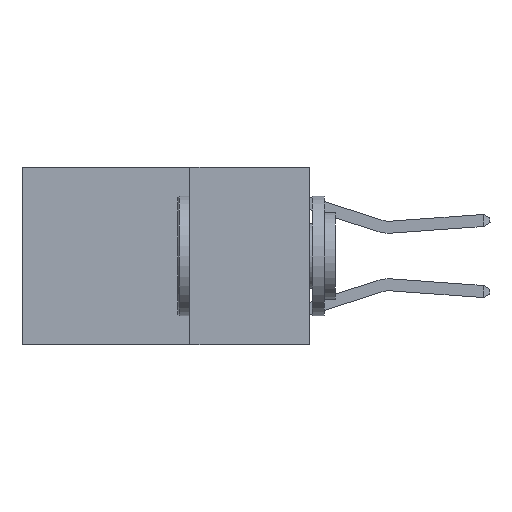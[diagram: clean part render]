
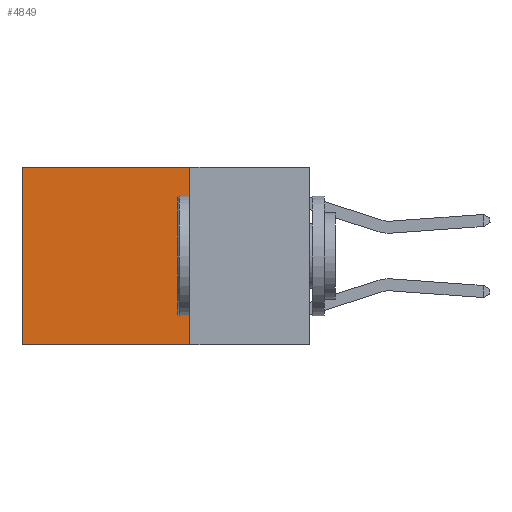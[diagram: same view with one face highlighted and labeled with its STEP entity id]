
A CAD part, left-side view. The second image highlights one B-rep face of the part: STEP entity #4849.
In plain terms, the highlighted planar face has unit normal (-1, 0, 0).
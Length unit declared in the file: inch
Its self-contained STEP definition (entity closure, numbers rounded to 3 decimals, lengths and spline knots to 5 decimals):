
#658 = VERTEX_POINT ( 'NONE', #7262 ) ;
#970 = VECTOR ( 'NONE', #3664, 39.37008 ) ;
#1154 = LINE ( 'NONE', #10167, #5738 ) ;
#1209 = VERTEX_POINT ( 'NONE', #4398 ) ;
#2331 = CARTESIAN_POINT ( 'NONE',  ( 0.2625, 0.25, 0. ) ) ;
#2369 = EDGE_CURVE ( 'NONE', #1209, #5428, #4144, .T. ) ;
#2580 = ORIENTED_EDGE ( 'NONE', *, *, #2369, .T. ) ;
#2636 = ORIENTED_EDGE ( 'NONE', *, *, #9742, .F. ) ;
#2655 = ORIENTED_EDGE ( 'NONE', *, *, #6685, .F. ) ;
#2946 = VERTEX_POINT ( 'NONE', #5557 ) ;
#2949 = ORIENTED_EDGE ( 'NONE', *, *, #4007, .T. ) ;
#3043 = CARTESIAN_POINT ( 'NONE',  ( 0.2625, 0.6, 0. ) ) ;
#3251 = PLANE ( 'NONE',  #6330 ) ;
#3318 = FACE_OUTER_BOUND ( 'NONE', #9757, .T. ) ;
#3664 = DIRECTION ( 'NONE',  ( 0., 0., -1. ) ) ;
#4007 = EDGE_CURVE ( 'NONE', #5428, #2946, #6175, .T. ) ;
#4144 = LINE ( 'NONE', #5724, #9201 ) ;
#4244 = CARTESIAN_POINT ( 'NONE',  ( 0.2625, 0.25, 0. ) ) ;
#4398 = CARTESIAN_POINT ( 'NONE',  ( 0.2625, 0.25, 0. ) ) ;
#4849 = ADVANCED_FACE ( 'NONE', ( #3318 ), #3251, .F. ) ;
#5181 = DIRECTION ( 'NONE',  ( 1., 0., 0. ) ) ;
#5428 = VERTEX_POINT ( 'NONE', #3043 ) ;
#5557 = CARTESIAN_POINT ( 'NONE',  ( 0.2625, 0.6, -0.37 ) ) ;
#5724 = CARTESIAN_POINT ( 'NONE',  ( 0.2625, 0.25, 0. ) ) ;
#5738 = VECTOR ( 'NONE', #10985, 39.37008 ) ;
#6175 = LINE ( 'NONE', #11529, #970 ) ;
#6235 = DIRECTION ( 'NONE',  ( 0., 0., -1. ) ) ;
#6264 = VECTOR ( 'NONE', #6235, 39.37008 ) ;
#6330 = AXIS2_PLACEMENT_3D ( 'NONE', #4244, #5181, #11194 ) ;
#6685 = EDGE_CURVE ( 'NONE', #658, #2946, #1154, .T. ) ;
#7262 = CARTESIAN_POINT ( 'NONE',  ( 0.2625, 0.25, -0.37 ) ) ;
#8572 = LINE ( 'NONE', #2331, #6264 ) ;
#9201 = VECTOR ( 'NONE', #11666, 39.37008 ) ;
#9742 = EDGE_CURVE ( 'NONE', #1209, #658, #8572, .T. ) ;
#9757 = EDGE_LOOP ( 'NONE', ( #2949, #2655, #2636, #2580 ) ) ;
#10167 = CARTESIAN_POINT ( 'NONE',  ( 0.2625, 0.25, -0.37 ) ) ;
#10985 = DIRECTION ( 'NONE',  ( 0., 1., 0. ) ) ;
#11194 = DIRECTION ( 'NONE',  ( 0., 0., -1. ) ) ;
#11529 = CARTESIAN_POINT ( 'NONE',  ( 0.2625, 0.6, 0. ) ) ;
#11666 = DIRECTION ( 'NONE',  ( 0., 1., 0. ) ) ;
